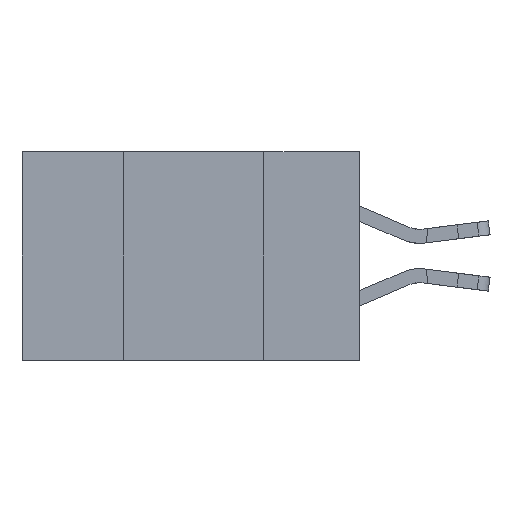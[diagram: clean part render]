
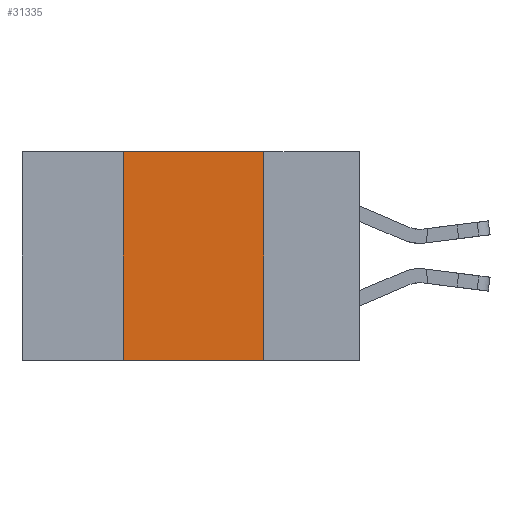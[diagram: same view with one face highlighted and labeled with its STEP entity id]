
A CAD part, left-side view. The second image highlights one B-rep face of the part: STEP entity #31335.
In plain terms, the highlighted planar face has unit normal (-1, 0, 0).
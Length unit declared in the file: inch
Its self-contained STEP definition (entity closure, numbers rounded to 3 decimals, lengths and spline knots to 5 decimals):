
#259 = LINE ( 'NONE', #25235, #18284 ) ;
#409 = DIRECTION ( 'NONE',  ( 0., 0., 1. ) ) ;
#755 = DIRECTION ( 'NONE',  ( 0., 0., -1. ) ) ;
#2370 = VECTOR ( 'NONE', #24269, 39.37008 ) ;
#2720 = LINE ( 'NONE', #15132, #22252 ) ;
#4539 = LINE ( 'NONE', #13310, #29828 ) ;
#5518 = CARTESIAN_POINT ( 'NONE',  ( 0., 0.17, -0.37 ) ) ;
#5536 = EDGE_CURVE ( 'NONE', #8675, #25679, #27794, .T. ) ;
#5627 = DIRECTION ( 'NONE',  ( 0., -1., 0. ) ) ;
#5944 = AXIS2_PLACEMENT_3D ( 'NONE', #28626, #16148, #755 ) ;
#6192 = EDGE_CURVE ( 'NONE', #8782, #6711, #2720, .T. ) ;
#6711 = VERTEX_POINT ( 'NONE', #9898 ) ;
#7134 = ORIENTED_EDGE ( 'NONE', *, *, #5536, .T. ) ;
#7165 = FACE_OUTER_BOUND ( 'NONE', #13778, .T. ) ;
#7443 = EDGE_CURVE ( 'NONE', #6711, #25679, #259, .T. ) ;
#8675 = VERTEX_POINT ( 'NONE', #17141 ) ;
#8782 = VERTEX_POINT ( 'NONE', #12551 ) ;
#9898 = CARTESIAN_POINT ( 'NONE',  ( 0., 0.17, 0. ) ) ;
#11110 = PLANE ( 'NONE',  #5944 ) ;
#12551 = CARTESIAN_POINT ( 'NONE',  ( 0., 0.42, 0. ) ) ;
#12736 = DIRECTION ( 'NONE',  ( 0., 0., -1. ) ) ;
#13310 = CARTESIAN_POINT ( 'NONE',  ( 0., 0.42, 0. ) ) ;
#13778 = EDGE_LOOP ( 'NONE', ( #15541, #23794, #31554, #7134 ) ) ;
#15132 = CARTESIAN_POINT ( 'NONE',  ( 0., 0.6, 0. ) ) ;
#15541 = ORIENTED_EDGE ( 'NONE', *, *, #7443, .F. ) ;
#16148 = DIRECTION ( 'NONE',  ( 1., 0., 0. ) ) ;
#17141 = CARTESIAN_POINT ( 'NONE',  ( 0., 0.42, -0.37 ) ) ;
#18284 = VECTOR ( 'NONE', #12736, 39.37008 ) ;
#19447 = CARTESIAN_POINT ( 'NONE',  ( 0., 0.6, -0.37 ) ) ;
#22252 = VECTOR ( 'NONE', #5627, 39.37008 ) ;
#23794 = ORIENTED_EDGE ( 'NONE', *, *, #6192, .F. ) ;
#24269 = DIRECTION ( 'NONE',  ( 0., -1., 0. ) ) ;
#25235 = CARTESIAN_POINT ( 'NONE',  ( 0., 0.17, 0. ) ) ;
#25679 = VERTEX_POINT ( 'NONE', #5518 ) ;
#27794 = LINE ( 'NONE', #19447, #2370 ) ;
#28611 = EDGE_CURVE ( 'NONE', #8675, #8782, #4539, .T. ) ;
#28626 = CARTESIAN_POINT ( 'NONE',  ( 0., 0.6, 0. ) ) ;
#29828 = VECTOR ( 'NONE', #409, 39.37008 ) ;
#31335 = ADVANCED_FACE ( 'NONE', ( #7165 ), #11110, .F. ) ;
#31554 = ORIENTED_EDGE ( 'NONE', *, *, #28611, .F. ) ;
